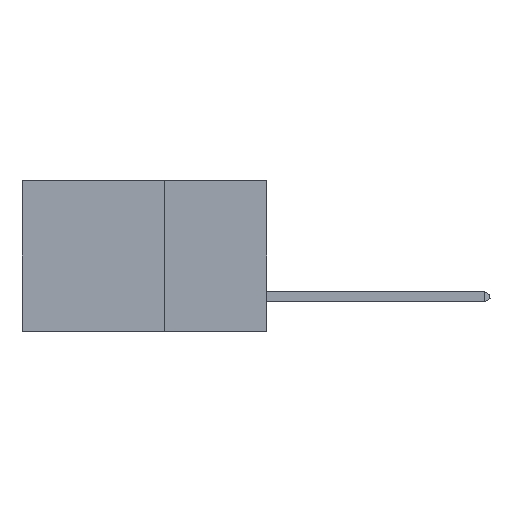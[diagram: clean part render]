
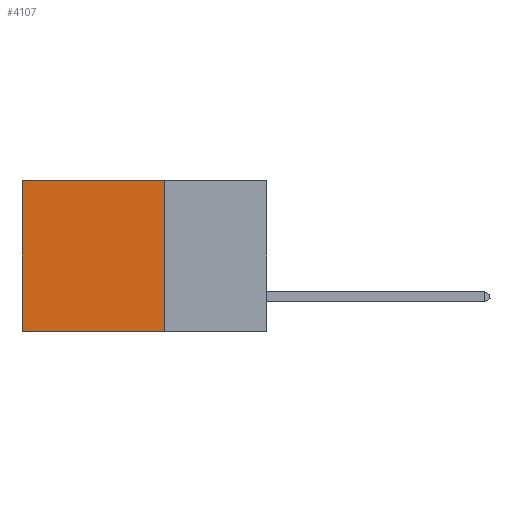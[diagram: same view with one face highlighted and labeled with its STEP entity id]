
A CAD part, left-side view. The second image highlights one B-rep face of the part: STEP entity #4107.
In plain terms, the highlighted planar face has unit normal (-1, 0, 0).
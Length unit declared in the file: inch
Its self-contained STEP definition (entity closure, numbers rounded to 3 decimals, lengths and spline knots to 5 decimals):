
#72 = EDGE_CURVE ( 'NONE', #5785, #4565, #3192, .T. ) ;
#470 = LINE ( 'NONE', #16145, #2418 ) ;
#974 = LINE ( 'NONE', #11004, #14397 ) ;
#1489 = EDGE_CURVE ( 'NONE', #3444, #5785, #974, .T. ) ;
#1519 = ORIENTED_EDGE ( 'NONE', *, *, #10544, .T. ) ;
#1613 = ORIENTED_EDGE ( 'NONE', *, *, #12954, .T. ) ;
#2418 = VECTOR ( 'NONE', #6630, 39.37008 ) ;
#2575 = AXIS2_PLACEMENT_3D ( 'NONE', #10096, #3174, #12833 ) ;
#2978 = ORIENTED_EDGE ( 'NONE', *, *, #1489, .F. ) ;
#3174 = DIRECTION ( 'NONE',  ( 1., 0., 0. ) ) ;
#3192 = LINE ( 'NONE', #14960, #12673 ) ;
#3444 = VERTEX_POINT ( 'NONE', #3718 ) ;
#3569 = VECTOR ( 'NONE', #8024, 39.37008 ) ;
#3718 = CARTESIAN_POINT ( 'NONE',  ( 0.2875, 0.25, 0. ) ) ;
#4107 = ADVANCED_FACE ( 'NONE', ( #13393 ), #14306, .F. ) ;
#4565 = VERTEX_POINT ( 'NONE', #10216 ) ;
#5451 = DIRECTION ( 'NONE',  ( 0., 0., -1. ) ) ;
#5785 = VERTEX_POINT ( 'NONE', #14706 ) ;
#6122 = CARTESIAN_POINT ( 'NONE',  ( 0.2875, 0.6, 0. ) ) ;
#6630 = DIRECTION ( 'NONE',  ( 0., 0., -1. ) ) ;
#6682 = CARTESIAN_POINT ( 'NONE',  ( 0.2875, 0.25, 0. ) ) ;
#8024 = DIRECTION ( 'NONE',  ( 0., 1., 0. ) ) ;
#9764 = VERTEX_POINT ( 'NONE', #6122 ) ;
#9793 = ORIENTED_EDGE ( 'NONE', *, *, #72, .F. ) ;
#10074 = LINE ( 'NONE', #6682, #3569 ) ;
#10096 = CARTESIAN_POINT ( 'NONE',  ( 0.2875, 0.25, 0. ) ) ;
#10216 = CARTESIAN_POINT ( 'NONE',  ( 0.2875, 0.6, -0.37 ) ) ;
#10544 = EDGE_CURVE ( 'NONE', #3444, #9764, #10074, .T. ) ;
#11004 = CARTESIAN_POINT ( 'NONE',  ( 0.2875, 0.25, 0. ) ) ;
#12673 = VECTOR ( 'NONE', #17839, 39.37008 ) ;
#12833 = DIRECTION ( 'NONE',  ( 0., 0., -1. ) ) ;
#12954 = EDGE_CURVE ( 'NONE', #9764, #4565, #470, .T. ) ;
#13393 = FACE_OUTER_BOUND ( 'NONE', #15070, .T. ) ;
#14306 = PLANE ( 'NONE',  #2575 ) ;
#14397 = VECTOR ( 'NONE', #5451, 39.37008 ) ;
#14706 = CARTESIAN_POINT ( 'NONE',  ( 0.2875, 0.25, -0.37 ) ) ;
#14960 = CARTESIAN_POINT ( 'NONE',  ( 0.2875, 0.25, -0.37 ) ) ;
#15070 = EDGE_LOOP ( 'NONE', ( #1613, #9793, #2978, #1519 ) ) ;
#16145 = CARTESIAN_POINT ( 'NONE',  ( 0.2875, 0.6, 0. ) ) ;
#17839 = DIRECTION ( 'NONE',  ( 0., 1., 0. ) ) ;
